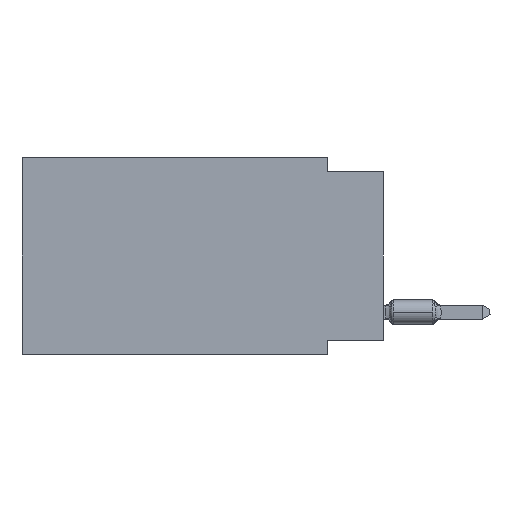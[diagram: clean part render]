
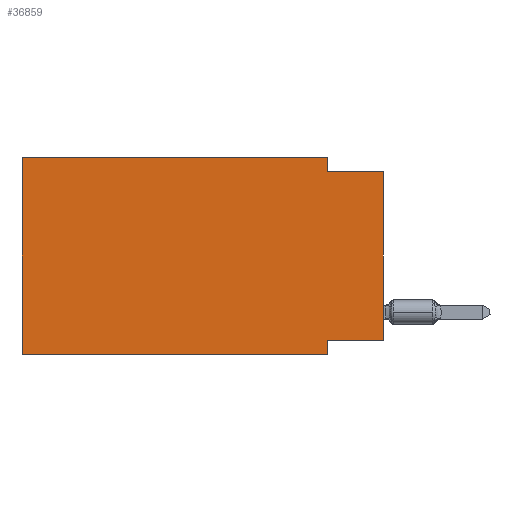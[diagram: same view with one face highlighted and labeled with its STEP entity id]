
A CAD part, left-side view. The second image highlights one B-rep face of the part: STEP entity #36859.
In plain terms, the highlighted planar face has unit normal (-1, 0, 0).
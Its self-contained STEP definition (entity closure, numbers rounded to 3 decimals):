
#2131 = DIRECTION ( 'NONE',  ( 0., 0., -1. ) ) ;
#2318 = DIRECTION ( 'NONE',  ( 0., -1., 0. ) ) ;
#3028 = LINE ( 'NONE', #11184, #14561 ) ;
#3389 = ORIENTED_EDGE ( 'NONE', *, *, #21581, .T. ) ;
#3749 = CARTESIAN_POINT ( 'NONE',  ( 0., 2.54, -8.255 ) ) ;
#4354 = VERTEX_POINT ( 'NONE', #3749 ) ;
#4869 = EDGE_CURVE ( 'NONE', #36994, #29134, #8398, .T. ) ;
#5530 = DIRECTION ( 'NONE',  ( 1., 0., 0. ) ) ;
#7742 = VECTOR ( 'NONE', #2318, 1000. ) ;
#8234 = LINE ( 'NONE', #11269, #21075 ) ;
#8380 = FACE_OUTER_BOUND ( 'NONE', #9258, .T. ) ;
#8398 = LINE ( 'NONE', #31399, #9099 ) ;
#8662 = ORIENTED_EDGE ( 'NONE', *, *, #4869, .F. ) ;
#9099 = VECTOR ( 'NONE', #2131, 1000. ) ;
#9258 = EDGE_LOOP ( 'NONE', ( #32599, #22184, #8662, #12852, #36952, #3389, #28712, #36454 ) ) ;
#9487 = VERTEX_POINT ( 'NONE', #27357 ) ;
#10428 = EDGE_CURVE ( 'NONE', #29134, #20042, #3028, .T. ) ;
#11184 = CARTESIAN_POINT ( 'NONE',  ( 0., 0., -0.635 ) ) ;
#11269 = CARTESIAN_POINT ( 'NONE',  ( 0., 16.383, 0. ) ) ;
#12624 = DIRECTION ( 'NONE',  ( 0., 0., -1. ) ) ;
#12691 = CARTESIAN_POINT ( 'NONE',  ( 0., 16.383, 0. ) ) ;
#12852 = ORIENTED_EDGE ( 'NONE', *, *, #24053, .F. ) ;
#12860 = LINE ( 'NONE', #35494, #20140 ) ;
#12962 = DIRECTION ( 'NONE',  ( 0., 1., 0. ) ) ;
#13161 = LINE ( 'NONE', #24401, #34128 ) ;
#13517 = LINE ( 'NONE', #24746, #16521 ) ;
#13634 = CARTESIAN_POINT ( 'NONE',  ( 0., 0., -8.255 ) ) ;
#14561 = VECTOR ( 'NONE', #28873, 1000. ) ;
#14582 = VERTEX_POINT ( 'NONE', #31114 ) ;
#16521 = VECTOR ( 'NONE', #12962, 1000. ) ;
#17106 = DIRECTION ( 'NONE',  ( 0., 0., -1. ) ) ;
#17868 = CARTESIAN_POINT ( 'NONE',  ( 0., 2.54, 0. ) ) ;
#19150 = VECTOR ( 'NONE', #32849, 1000. ) ;
#19951 = PLANE ( 'NONE',  #26771 ) ;
#20042 = VERTEX_POINT ( 'NONE', #20448 ) ;
#20140 = VECTOR ( 'NONE', #30340, 1000. ) ;
#20175 = VERTEX_POINT ( 'NONE', #35467 ) ;
#20448 = CARTESIAN_POINT ( 'NONE',  ( 0., 0., -0.635 ) ) ;
#21075 = VECTOR ( 'NONE', #31614, 1000. ) ;
#21581 = EDGE_CURVE ( 'NONE', #9487, #20175, #22449, .T. ) ;
#21741 = CARTESIAN_POINT ( 'NONE',  ( 0., 16.383, 0. ) ) ;
#22184 = ORIENTED_EDGE ( 'NONE', *, *, #10428, .F. ) ;
#22449 = LINE ( 'NONE', #28355, #7742 ) ;
#23203 = EDGE_CURVE ( 'NONE', #9487, #14582, #30002, .T. ) ;
#23340 = CARTESIAN_POINT ( 'NONE',  ( 0., 2.54, -0.635 ) ) ;
#24053 = EDGE_CURVE ( 'NONE', #14582, #36994, #8234, .T. ) ;
#24401 = CARTESIAN_POINT ( 'NONE',  ( 0., 2.54, -8.89 ) ) ;
#24746 = CARTESIAN_POINT ( 'NONE',  ( 0., 0., -8.255 ) ) ;
#26771 = AXIS2_PLACEMENT_3D ( 'NONE', #21741, #5530, #17106 ) ;
#27357 = CARTESIAN_POINT ( 'NONE',  ( 0., 16.383, -8.89 ) ) ;
#28355 = CARTESIAN_POINT ( 'NONE',  ( 0., 16.383, -8.89 ) ) ;
#28712 = ORIENTED_EDGE ( 'NONE', *, *, #34804, .F. ) ;
#28873 = DIRECTION ( 'NONE',  ( 0., -1., 0. ) ) ;
#29134 = VERTEX_POINT ( 'NONE', #23340 ) ;
#29266 = EDGE_CURVE ( 'NONE', #36029, #20042, #12860, .T. ) ;
#30002 = LINE ( 'NONE', #12691, #19150 ) ;
#30167 = EDGE_CURVE ( 'NONE', #36029, #4354, #13517, .T. ) ;
#30340 = DIRECTION ( 'NONE',  ( 0., 0., 1. ) ) ;
#31114 = CARTESIAN_POINT ( 'NONE',  ( 0., 16.383, 0. ) ) ;
#31399 = CARTESIAN_POINT ( 'NONE',  ( 0., 2.54, 0. ) ) ;
#31614 = DIRECTION ( 'NONE',  ( 0., -1., 0. ) ) ;
#32599 = ORIENTED_EDGE ( 'NONE', *, *, #29266, .T. ) ;
#32849 = DIRECTION ( 'NONE',  ( 0., 0., 1. ) ) ;
#34128 = VECTOR ( 'NONE', #12624, 1000. ) ;
#34804 = EDGE_CURVE ( 'NONE', #4354, #20175, #13161, .T. ) ;
#35467 = CARTESIAN_POINT ( 'NONE',  ( 0., 2.54, -8.89 ) ) ;
#35494 = CARTESIAN_POINT ( 'NONE',  ( 0., 0., 0. ) ) ;
#36029 = VERTEX_POINT ( 'NONE', #13634 ) ;
#36454 = ORIENTED_EDGE ( 'NONE', *, *, #30167, .F. ) ;
#36859 = ADVANCED_FACE ( 'NONE', ( #8380 ), #19951, .F. ) ;
#36952 = ORIENTED_EDGE ( 'NONE', *, *, #23203, .F. ) ;
#36994 = VERTEX_POINT ( 'NONE', #17868 ) ;
